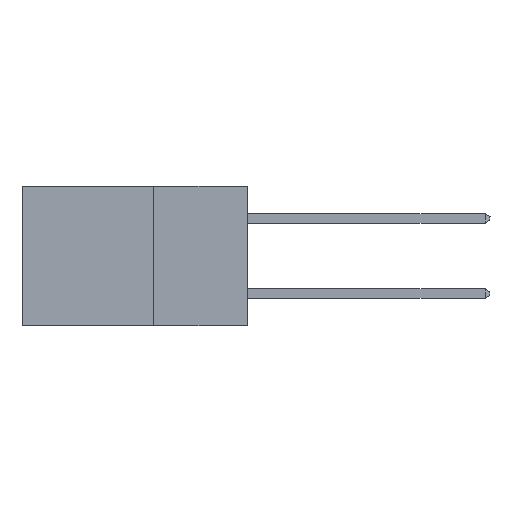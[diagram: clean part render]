
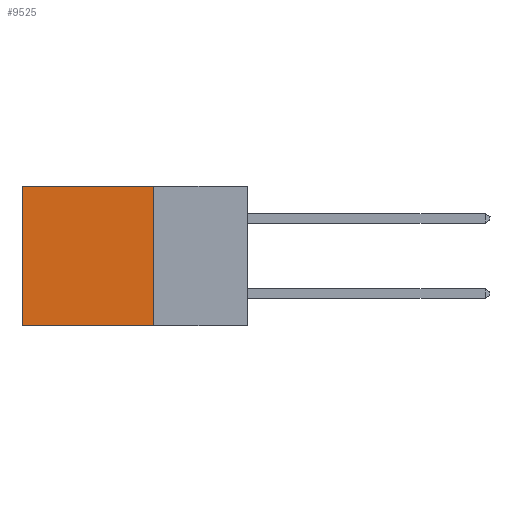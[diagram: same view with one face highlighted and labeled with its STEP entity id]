
A CAD part, left-side view. The second image highlights one B-rep face of the part: STEP entity #9525.
In plain terms, the highlighted planar face has unit normal (-1, 0, 0).
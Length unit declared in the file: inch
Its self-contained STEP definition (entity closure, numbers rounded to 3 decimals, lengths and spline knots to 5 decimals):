
#257 = CARTESIAN_POINT ( 'NONE',  ( 0.2615, 0.6, -0.37 ) ) ;
#533 = DIRECTION ( 'NONE',  ( 0., 1., 0. ) ) ;
#898 = LINE ( 'NONE', #3785, #17052 ) ;
#1583 = CARTESIAN_POINT ( 'NONE',  ( 0.2615, 0.6, 0. ) ) ;
#2443 = ORIENTED_EDGE ( 'NONE', *, *, #12300, .T. ) ;
#3044 = DIRECTION ( 'NONE',  ( 0., 0., -1. ) ) ;
#3599 = VERTEX_POINT ( 'NONE', #1583 ) ;
#3785 = CARTESIAN_POINT ( 'NONE',  ( 0.2615, 0.25, -0.37 ) ) ;
#3826 = VECTOR ( 'NONE', #10693, 39.37008 ) ;
#4279 = DIRECTION ( 'NONE',  ( 0., 0., -1. ) ) ;
#4629 = LINE ( 'NONE', #257, #12693 ) ;
#6294 = EDGE_LOOP ( 'NONE', ( #2443, #15514, #9257, #16885 ) ) ;
#6303 = EDGE_CURVE ( 'NONE', #14446, #13165, #6798, .T. ) ;
#6728 = AXIS2_PLACEMENT_3D ( 'NONE', #15240, #16461, #10797 ) ;
#6798 = LINE ( 'NONE', #8288, #17310 ) ;
#6805 = FACE_OUTER_BOUND ( 'NONE', #6294, .T. ) ;
#8288 = CARTESIAN_POINT ( 'NONE',  ( 0.2615, 0.25, -0.37 ) ) ;
#8389 = EDGE_CURVE ( 'NONE', #13165, #10317, #898, .T. ) ;
#9257 = ORIENTED_EDGE ( 'NONE', *, *, #6303, .F. ) ;
#9525 = ADVANCED_FACE ( 'NONE', ( #6805 ), #13664, .F. ) ;
#10317 = VERTEX_POINT ( 'NONE', #11440 ) ;
#10693 = DIRECTION ( 'NONE',  ( 0., 1., 0. ) ) ;
#10797 = DIRECTION ( 'NONE',  ( 0., 0., -1. ) ) ;
#11440 = CARTESIAN_POINT ( 'NONE',  ( 0.2615, 0.6, -0.37 ) ) ;
#11703 = CARTESIAN_POINT ( 'NONE',  ( 0.2615, 0.25, -0.37 ) ) ;
#11909 = CARTESIAN_POINT ( 'NONE',  ( 0.2615, 0.25, 0. ) ) ;
#12300 = EDGE_CURVE ( 'NONE', #3599, #10317, #4629, .T. ) ;
#12693 = VECTOR ( 'NONE', #3044, 39.37008 ) ;
#13165 = VERTEX_POINT ( 'NONE', #11703 ) ;
#13644 = LINE ( 'NONE', #13737, #3826 ) ;
#13664 = PLANE ( 'NONE',  #6728 ) ;
#13737 = CARTESIAN_POINT ( 'NONE',  ( 0.2615, 0.25, 0. ) ) ;
#14446 = VERTEX_POINT ( 'NONE', #11909 ) ;
#14620 = EDGE_CURVE ( 'NONE', #14446, #3599, #13644, .T. ) ;
#15240 = CARTESIAN_POINT ( 'NONE',  ( 0.2615, 0.25, -0.37 ) ) ;
#15514 = ORIENTED_EDGE ( 'NONE', *, *, #8389, .F. ) ;
#16461 = DIRECTION ( 'NONE',  ( 1., 0., 0. ) ) ;
#16885 = ORIENTED_EDGE ( 'NONE', *, *, #14620, .T. ) ;
#17052 = VECTOR ( 'NONE', #533, 39.37008 ) ;
#17310 = VECTOR ( 'NONE', #4279, 39.37008 ) ;
